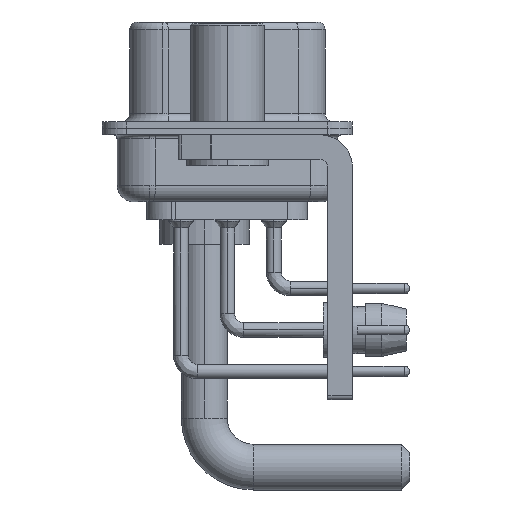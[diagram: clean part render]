
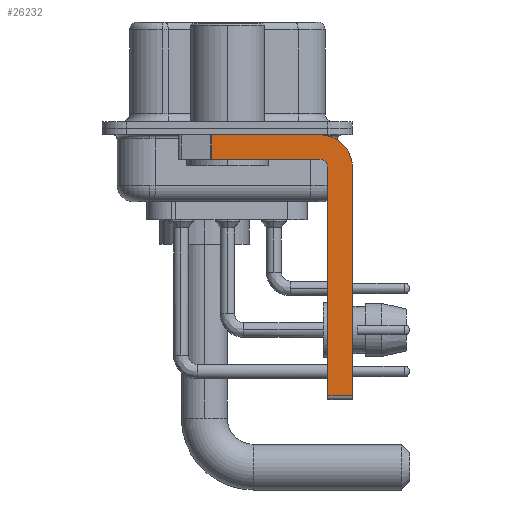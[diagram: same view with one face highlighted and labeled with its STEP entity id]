
A CAD part, left-side view. The second image highlights one B-rep face of the part: STEP entity #26232.
In plain terms, the highlighted planar face has unit normal (-1, 0, 0).
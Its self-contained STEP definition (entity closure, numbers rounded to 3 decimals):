
#87 = CARTESIAN_POINT ( 'NONE',  ( -2.9, -6.15, -2.4 ) ) ;
#1854 = VERTEX_POINT ( 'NONE', #26539 ) ;
#2632 = EDGE_CURVE ( 'NONE', #1854, #11808, #32906, .T. ) ;
#2699 = CARTESIAN_POINT ( 'NONE',  ( -2.9, -5.65, -2.4 ) ) ;
#3311 = PLANE ( 'NONE',  #30344 ) ;
#3487 = ORIENTED_EDGE ( 'NONE', *, *, #30502, .F. ) ;
#3553 = CARTESIAN_POINT ( 'NONE',  ( -2.9, -7.65, -16.35 ) ) ;
#3719 = CIRCLE ( 'NONE', #21975, 0.5 ) ;
#4134 = AXIS2_PLACEMENT_3D ( 'NONE', #28432, #6475, #15257 ) ;
#5833 = CARTESIAN_POINT ( 'NONE',  ( -2.9, -5.65, -1.9 ) ) ;
#5961 = DIRECTION ( 'NONE',  ( 1., 0., 0. ) ) ;
#6475 = DIRECTION ( 'NONE',  ( 1., 0., 0. ) ) ;
#7332 = DIRECTION ( 'NONE',  ( 0., 0., -1. ) ) ;
#7606 = DIRECTION ( 'NONE',  ( 0., -1., 0. ) ) ;
#8039 = CARTESIAN_POINT ( 'NONE',  ( -2.9, 0.978, -1.9 ) ) ;
#8647 = LINE ( 'NONE', #8039, #28778 ) ;
#9207 = CARTESIAN_POINT ( 'NONE',  ( -2.9, 0.978, -0.4 ) ) ;
#9394 = DIRECTION ( 'NONE',  ( 0., 0., -1. ) ) ;
#9431 = DIRECTION ( 'NONE',  ( 0., 0., -1. ) ) ;
#10011 = EDGE_CURVE ( 'NONE', #26142, #30116, #8647, .T. ) ;
#11479 = LINE ( 'NONE', #23919, #20708 ) ;
#11808 = VERTEX_POINT ( 'NONE', #25353 ) ;
#12558 = CARTESIAN_POINT ( 'NONE',  ( -2.9, 0.978, -1.9 ) ) ;
#13005 = LINE ( 'NONE', #22789, #16362 ) ;
#15257 = DIRECTION ( 'NONE',  ( 0., 0., -1. ) ) ;
#15869 = DIRECTION ( 'NONE',  ( 0., 1., 0. ) ) ;
#15912 = VECTOR ( 'NONE', #21072, 1000. ) ;
#15932 = DIRECTION ( 'NONE',  ( 0., -1., 0. ) ) ;
#16362 = VECTOR ( 'NONE', #15869, 1000. ) ;
#16919 = VECTOR ( 'NONE', #15932, 1000. ) ;
#18997 = CARTESIAN_POINT ( 'NONE',  ( -2.9, -5.65, -16.35 ) ) ;
#19650 = CARTESIAN_POINT ( 'NONE',  ( -2.9, -6.15, -16.35 ) ) ;
#19834 = EDGE_CURVE ( 'NONE', #26142, #1854, #11479, .T. ) ;
#20708 = VECTOR ( 'NONE', #7606, 1000. ) ;
#20871 = LINE ( 'NONE', #36613, #15912 ) ;
#21071 = ORIENTED_EDGE ( 'NONE', *, *, #19834, .F. ) ;
#21072 = DIRECTION ( 'NONE',  ( 0., 0., 1. ) ) ;
#21354 = EDGE_CURVE ( 'NONE', #35454, #39985, #32267, .T. ) ;
#21975 = AXIS2_PLACEMENT_3D ( 'NONE', #26105, #23237, #38182 ) ;
#22635 = CARTESIAN_POINT ( 'NONE',  ( -2.9, -7.65, -2.4 ) ) ;
#22789 = CARTESIAN_POINT ( 'NONE',  ( -2.9, -5.65, -1.9 ) ) ;
#22863 = EDGE_CURVE ( 'NONE', #23254, #30116, #13005, .T. ) ;
#23237 = DIRECTION ( 'NONE',  ( -1., 0., 0. ) ) ;
#23254 = VERTEX_POINT ( 'NONE', #5833 ) ;
#23615 = ORIENTED_EDGE ( 'NONE', *, *, #40295, .F. ) ;
#23919 = CARTESIAN_POINT ( 'NONE',  ( -2.9, 3., -0.4 ) ) ;
#25353 = CARTESIAN_POINT ( 'NONE',  ( -2.9, -7.65, -2.4 ) ) ;
#25507 = LINE ( 'NONE', #22635, #32566 ) ;
#26105 = CARTESIAN_POINT ( 'NONE',  ( -2.9, -5.65, -2.4 ) ) ;
#26142 = VERTEX_POINT ( 'NONE', #9207 ) ;
#26196 = ORIENTED_EDGE ( 'NONE', *, *, #10011, .T. ) ;
#26232 = ADVANCED_FACE ( 'NONE', ( #28367 ), #3311, .F. ) ;
#26539 = CARTESIAN_POINT ( 'NONE',  ( -2.9, -5.65, -0.4 ) ) ;
#28145 = EDGE_CURVE ( 'NONE', #38664, #23254, #3719, .T. ) ;
#28367 = FACE_OUTER_BOUND ( 'NONE', #35813, .T. ) ;
#28432 = CARTESIAN_POINT ( 'NONE',  ( -2.9, -5.65, -2.4 ) ) ;
#28778 = VECTOR ( 'NONE', #9394, 1000. ) ;
#29260 = ORIENTED_EDGE ( 'NONE', *, *, #21354, .T. ) ;
#30116 = VERTEX_POINT ( 'NONE', #12558 ) ;
#30344 = AXIS2_PLACEMENT_3D ( 'NONE', #2699, #5961, #9431 ) ;
#30502 = EDGE_CURVE ( 'NONE', #11808, #39985, #25507, .T. ) ;
#31870 = ORIENTED_EDGE ( 'NONE', *, *, #28145, .F. ) ;
#32267 = LINE ( 'NONE', #18997, #16919 ) ;
#32566 = VECTOR ( 'NONE', #7332, 1000. ) ;
#32906 = CIRCLE ( 'NONE', #4134, 2. ) ;
#35454 = VERTEX_POINT ( 'NONE', #19650 ) ;
#35813 = EDGE_LOOP ( 'NONE', ( #21071, #26196, #39456, #31870, #23615, #29260, #3487, #35981 ) ) ;
#35981 = ORIENTED_EDGE ( 'NONE', *, *, #2632, .F. ) ;
#36613 = CARTESIAN_POINT ( 'NONE',  ( -2.9, -6.15, -16.6 ) ) ;
#38182 = DIRECTION ( 'NONE',  ( 0., 0., 1. ) ) ;
#38664 = VERTEX_POINT ( 'NONE', #87 ) ;
#39456 = ORIENTED_EDGE ( 'NONE', *, *, #22863, .F. ) ;
#39985 = VERTEX_POINT ( 'NONE', #3553 ) ;
#40295 = EDGE_CURVE ( 'NONE', #35454, #38664, #20871, .T. ) ;
